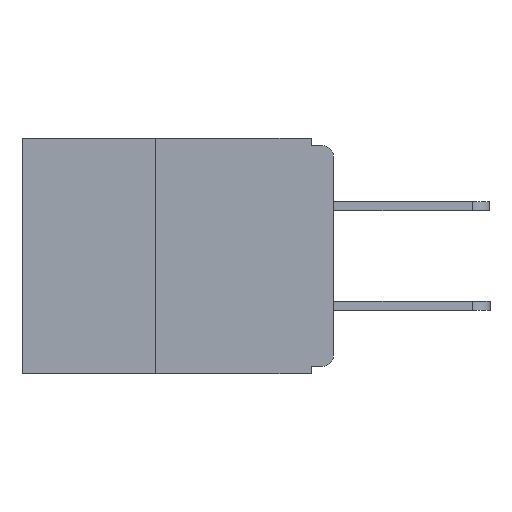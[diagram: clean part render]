
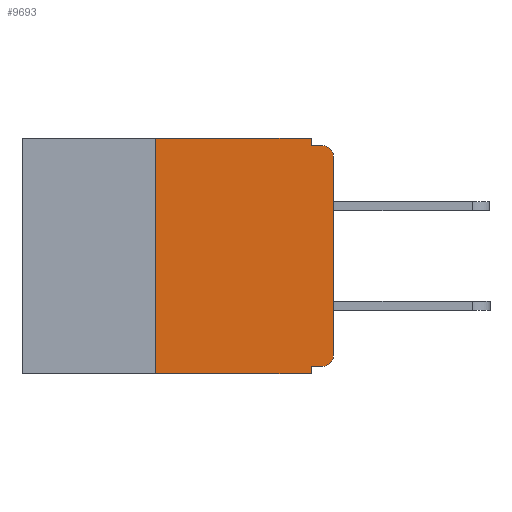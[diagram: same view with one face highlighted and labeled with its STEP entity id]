
A CAD part, left-side view. The second image highlights one B-rep face of the part: STEP entity #9693.
In plain terms, the highlighted planar face has unit normal (-1, 0, 0).
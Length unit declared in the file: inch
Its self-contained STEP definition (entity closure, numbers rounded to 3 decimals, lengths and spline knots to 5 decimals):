
#14 = DIRECTION ( 'NONE',  ( 0., -1., 0. ) ) ;
#39 = CARTESIAN_POINT ( 'NONE',  ( 0., 0.015, -0.01 ) ) ;
#113 = VERTEX_POINT ( 'NONE', #15634 ) ;
#186 = ORIENTED_EDGE ( 'NONE', *, *, #2726, .T. ) ;
#938 = CARTESIAN_POINT ( 'NONE',  ( 0., 0.031, 0. ) ) ;
#1004 = VERTEX_POINT ( 'NONE', #16852 ) ;
#1579 = ORIENTED_EDGE ( 'NONE', *, *, #3151, .F. ) ;
#1816 = CARTESIAN_POINT ( 'NONE',  ( 0., 0.25, -0.33 ) ) ;
#1950 = VECTOR ( 'NONE', #17890, 39.37008 ) ;
#2436 = LINE ( 'NONE', #14081, #18005 ) ;
#2573 = CIRCLE ( 'NONE', #3453, 0.015 ) ;
#2674 = CARTESIAN_POINT ( 'NONE',  ( 0., 0.015, -0.32 ) ) ;
#2726 = EDGE_CURVE ( 'NONE', #1004, #17519, #6363, .T. ) ;
#2989 = VECTOR ( 'NONE', #10893, 39.37008 ) ;
#3151 = EDGE_CURVE ( 'NONE', #18299, #10111, #15089, .T. ) ;
#3175 = ORIENTED_EDGE ( 'NONE', *, *, #9569, .F. ) ;
#3399 = LINE ( 'NONE', #16862, #18774 ) ;
#3453 = AXIS2_PLACEMENT_3D ( 'NONE', #6246, #6179, #6113 ) ;
#3528 = LINE ( 'NONE', #7299, #14636 ) ;
#4258 = EDGE_CURVE ( 'NONE', #5216, #1004, #16898, .T. ) ;
#4622 = CARTESIAN_POINT ( 'NONE',  ( 0., 0.031, 0. ) ) ;
#4645 = DIRECTION ( 'NONE',  ( 0., 0., -1. ) ) ;
#4706 = DIRECTION ( 'NONE',  ( 0., 0., -1. ) ) ;
#4730 = CARTESIAN_POINT ( 'NONE',  ( 0., 0.031, -0.33 ) ) ;
#5056 = LINE ( 'NONE', #4622, #9112 ) ;
#5135 = LINE ( 'NONE', #19205, #5652 ) ;
#5216 = VERTEX_POINT ( 'NONE', #2674 ) ;
#5345 = FACE_OUTER_BOUND ( 'NONE', #13442, .T. ) ;
#5652 = VECTOR ( 'NONE', #19400, 39.37008 ) ;
#5677 = DIRECTION ( 'NONE',  ( 0., 0., -1. ) ) ;
#5697 = DIRECTION ( 'NONE',  ( 1., 0., 0. ) ) ;
#5717 = CARTESIAN_POINT ( 'NONE',  ( 0., 0.437, 0. ) ) ;
#5742 = PLANE ( 'NONE',  #11013 ) ;
#6113 = DIRECTION ( 'NONE',  ( 0., 0., -1. ) ) ;
#6179 = DIRECTION ( 'NONE',  ( -1., 0., 0. ) ) ;
#6219 = CARTESIAN_POINT ( 'NONE',  ( 0., 0.031, -0.01 ) ) ;
#6246 = CARTESIAN_POINT ( 'NONE',  ( 0., 0.015, -0.025 ) ) ;
#6363 = LINE ( 'NONE', #18345, #1950 ) ;
#6660 = ORIENTED_EDGE ( 'NONE', *, *, #10444, .F. ) ;
#6853 = CARTESIAN_POINT ( 'NONE',  ( 0., 0.015, -0.305 ) ) ;
#6862 = ORIENTED_EDGE ( 'NONE', *, *, #7545, .F. ) ;
#7225 = CARTESIAN_POINT ( 'NONE',  ( 0., 0.437, 0. ) ) ;
#7299 = CARTESIAN_POINT ( 'NONE',  ( 0., 0.25, -0.33 ) ) ;
#7359 = DIRECTION ( 'NONE',  ( 0., 0., 1. ) ) ;
#7439 = EDGE_CURVE ( 'NONE', #17519, #10173, #2573, .T. ) ;
#7545 = EDGE_CURVE ( 'NONE', #113, #19030, #18335, .T. ) ;
#7815 = CARTESIAN_POINT ( 'NONE',  ( 0., 0., -0.025 ) ) ;
#8474 = ORIENTED_EDGE ( 'NONE', *, *, #15309, .F. ) ;
#8524 = CARTESIAN_POINT ( 'NONE',  ( 0., 0.25, 0. ) ) ;
#8555 = EDGE_CURVE ( 'NONE', #19287, #19030, #5135, .T. ) ;
#8803 = DIRECTION ( 'NONE',  ( 0., 0., -1. ) ) ;
#8869 = DIRECTION ( 'NONE',  ( -1., 0., 0. ) ) ;
#9055 = CARTESIAN_POINT ( 'NONE',  ( 0., 0.031, -0.33 ) ) ;
#9112 = VECTOR ( 'NONE', #4645, 39.37008 ) ;
#9569 = EDGE_CURVE ( 'NONE', #19287, #18299, #3528, .T. ) ;
#9693 = ADVANCED_FACE ( 'NONE', ( #5345 ), #5742, .F. ) ;
#10111 = VERTEX_POINT ( 'NONE', #938 ) ;
#10173 = VERTEX_POINT ( 'NONE', #39 ) ;
#10444 = EDGE_CURVE ( 'NONE', #5216, #113, #2436, .T. ) ;
#10893 = DIRECTION ( 'NONE',  ( 0., -1., 0. ) ) ;
#11013 = AXIS2_PLACEMENT_3D ( 'NONE', #5717, #5697, #5677 ) ;
#11109 = ORIENTED_EDGE ( 'NONE', *, *, #4258, .T. ) ;
#12560 = EDGE_CURVE ( 'NONE', #10111, #14481, #5056, .T. ) ;
#13442 = EDGE_LOOP ( 'NONE', ( #186, #18263, #8474, #16477, #1579, #3175, #14243, #6862, #6660, #11109 ) ) ;
#14018 = DIRECTION ( 'NONE',  ( 0., 1., 0. ) ) ;
#14081 = CARTESIAN_POINT ( 'NONE',  ( 0., 0., -0.32 ) ) ;
#14243 = ORIENTED_EDGE ( 'NONE', *, *, #8555, .T. ) ;
#14481 = VERTEX_POINT ( 'NONE', #6219 ) ;
#14636 = VECTOR ( 'NONE', #7359, 39.37008 ) ;
#15089 = LINE ( 'NONE', #7225, #2989 ) ;
#15309 = EDGE_CURVE ( 'NONE', #14481, #10173, #3399, .T. ) ;
#15634 = CARTESIAN_POINT ( 'NONE',  ( 0., 0.031, -0.32 ) ) ;
#16477 = ORIENTED_EDGE ( 'NONE', *, *, #12560, .F. ) ;
#16852 = CARTESIAN_POINT ( 'NONE',  ( 0., 0., -0.305 ) ) ;
#16862 = CARTESIAN_POINT ( 'NONE',  ( 0., 0., -0.01 ) ) ;
#16898 = CIRCLE ( 'NONE', #17607, 0.015 ) ;
#17519 = VERTEX_POINT ( 'NONE', #7815 ) ;
#17607 = AXIS2_PLACEMENT_3D ( 'NONE', #6853, #8869, #8803 ) ;
#17890 = DIRECTION ( 'NONE',  ( 0., 0., 1. ) ) ;
#18005 = VECTOR ( 'NONE', #14018, 39.37008 ) ;
#18263 = ORIENTED_EDGE ( 'NONE', *, *, #7439, .T. ) ;
#18299 = VERTEX_POINT ( 'NONE', #8524 ) ;
#18335 = LINE ( 'NONE', #4730, #19177 ) ;
#18345 = CARTESIAN_POINT ( 'NONE',  ( 0., 0., 0. ) ) ;
#18774 = VECTOR ( 'NONE', #14, 39.37008 ) ;
#19030 = VERTEX_POINT ( 'NONE', #9055 ) ;
#19177 = VECTOR ( 'NONE', #4706, 39.37008 ) ;
#19205 = CARTESIAN_POINT ( 'NONE',  ( 0., 0.437, -0.33 ) ) ;
#19287 = VERTEX_POINT ( 'NONE', #1816 ) ;
#19400 = DIRECTION ( 'NONE',  ( 0., -1., 0. ) ) ;
